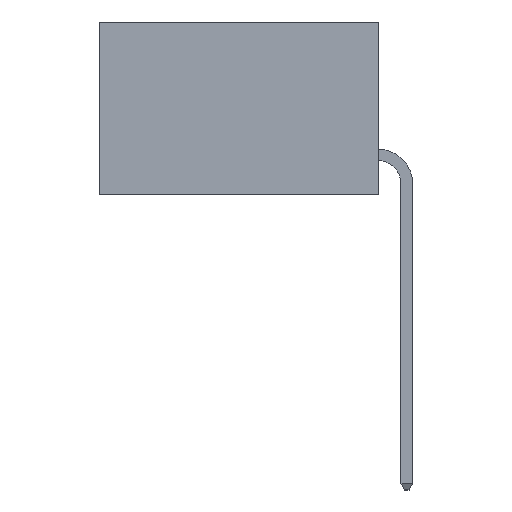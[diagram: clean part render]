
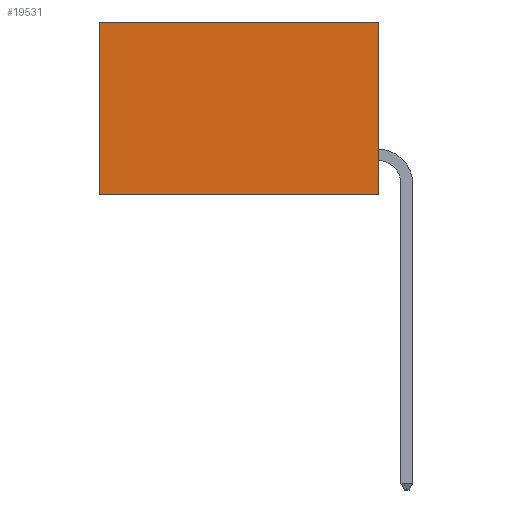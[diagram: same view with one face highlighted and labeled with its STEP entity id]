
A CAD part, left-side view. The second image highlights one B-rep face of the part: STEP entity #19531.
In plain terms, the highlighted planar face has unit normal (-1, 0, 0).
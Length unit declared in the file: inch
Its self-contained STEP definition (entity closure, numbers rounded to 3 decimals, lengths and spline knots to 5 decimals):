
#121 = VERTEX_POINT ( 'NONE', #20584 ) ;
#598 = ORIENTED_EDGE ( 'NONE', *, *, #4375, .T. ) ;
#898 = CARTESIAN_POINT ( 'NONE',  ( 0.2615, 0., 0. ) ) ;
#1121 = VERTEX_POINT ( 'NONE', #898 ) ;
#1771 = EDGE_LOOP ( 'NONE', ( #598, #16259, #6625, #3960 ) ) ;
#1809 = CARTESIAN_POINT ( 'NONE',  ( 0.2615, 0., -0.37 ) ) ;
#3960 = ORIENTED_EDGE ( 'NONE', *, *, #17770, .T. ) ;
#4375 = EDGE_CURVE ( 'NONE', #11059, #121, #7175, .T. ) ;
#4853 = PLANE ( 'NONE',  #17743 ) ;
#5195 = CARTESIAN_POINT ( 'NONE',  ( 0.2615, 0., 0. ) ) ;
#5422 = LINE ( 'NONE', #5195, #14471 ) ;
#6103 = VECTOR ( 'NONE', #24073, 39.37008 ) ;
#6574 = FACE_OUTER_BOUND ( 'NONE', #1771, .T. ) ;
#6625 = ORIENTED_EDGE ( 'NONE', *, *, #7536, .F. ) ;
#6843 = DIRECTION ( 'NONE',  ( 1., 0., 0. ) ) ;
#7175 = LINE ( 'NONE', #9179, #16730 ) ;
#7536 = EDGE_CURVE ( 'NONE', #1121, #11710, #13951, .T. ) ;
#7573 = CARTESIAN_POINT ( 'NONE',  ( 0.2615, 0.6, 0. ) ) ;
#8513 = DIRECTION ( 'NONE',  ( 0., 0., -1. ) ) ;
#8818 = VECTOR ( 'NONE', #12922, 39.37008 ) ;
#9179 = CARTESIAN_POINT ( 'NONE',  ( 0.2615, 0.6, -0.37 ) ) ;
#11059 = VERTEX_POINT ( 'NONE', #7573 ) ;
#11285 = LINE ( 'NONE', #22195, #6103 ) ;
#11710 = VERTEX_POINT ( 'NONE', #1809 ) ;
#12694 = CARTESIAN_POINT ( 'NONE',  ( 0.2615, 0., -0.37 ) ) ;
#12922 = DIRECTION ( 'NONE',  ( 0., 0., -1. ) ) ;
#13951 = LINE ( 'NONE', #12694, #8818 ) ;
#14471 = VECTOR ( 'NONE', #20454, 39.37008 ) ;
#15159 = EDGE_CURVE ( 'NONE', #11710, #121, #11285, .T. ) ;
#16259 = ORIENTED_EDGE ( 'NONE', *, *, #15159, .F. ) ;
#16378 = CARTESIAN_POINT ( 'NONE',  ( 0.2615, 0., -0.37 ) ) ;
#16730 = VECTOR ( 'NONE', #8513, 39.37008 ) ;
#17743 = AXIS2_PLACEMENT_3D ( 'NONE', #16378, #6843, #20138 ) ;
#17770 = EDGE_CURVE ( 'NONE', #1121, #11059, #5422, .T. ) ;
#19531 = ADVANCED_FACE ( 'NONE', ( #6574 ), #4853, .F. ) ;
#20138 = DIRECTION ( 'NONE',  ( 0., 0., -1. ) ) ;
#20454 = DIRECTION ( 'NONE',  ( 0., 1., 0. ) ) ;
#20584 = CARTESIAN_POINT ( 'NONE',  ( 0.2615, 0.6, -0.37 ) ) ;
#22195 = CARTESIAN_POINT ( 'NONE',  ( 0.2615, 0., -0.37 ) ) ;
#24073 = DIRECTION ( 'NONE',  ( 0., 1., 0. ) ) ;
